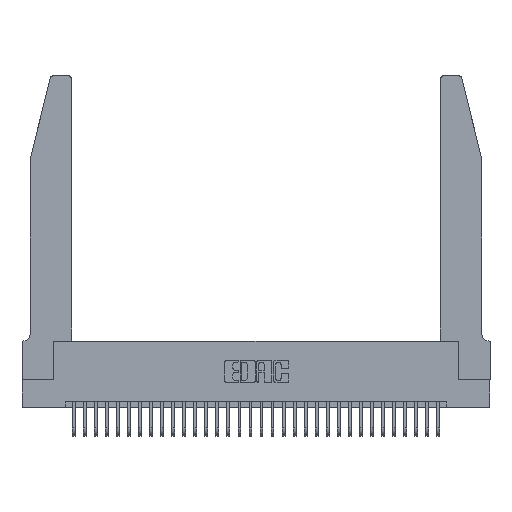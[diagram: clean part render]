
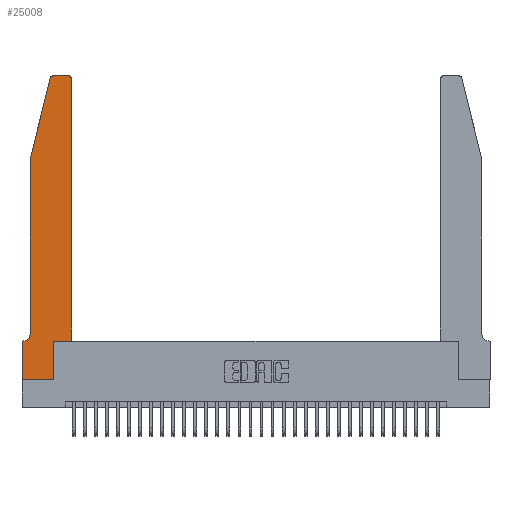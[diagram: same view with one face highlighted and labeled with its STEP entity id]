
A CAD part, top view. The second image highlights one B-rep face of the part: STEP entity #25008.
In plain terms, the highlighted planar face has unit normal (0, 0, 1).
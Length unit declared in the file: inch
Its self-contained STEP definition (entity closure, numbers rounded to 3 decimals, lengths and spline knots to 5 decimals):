
#383 = VECTOR ( 'NONE', #31586, 39.37008 ) ;
#1047 = VECTOR ( 'NONE', #8465, 39.37008 ) ;
#1479 = ORIENTED_EDGE ( 'NONE', *, *, #18732, .T. ) ;
#1792 = CARTESIAN_POINT ( 'NONE',  ( 0.2865, 0.35, 0.37 ) ) ;
#1865 = DIRECTION ( 'NONE',  ( 0., 0., 1. ) ) ;
#2459 = CARTESIAN_POINT ( 'NONE',  ( 0.4205, 2.75, 0.37 ) ) ;
#2580 = VECTOR ( 'NONE', #15802, 39.37008 ) ;
#2673 = ORIENTED_EDGE ( 'NONE', *, *, #33491, .T. ) ;
#2712 = CARTESIAN_POINT ( 'NONE',  ( 0.4505, 0.35, 0.37 ) ) ;
#3021 = CARTESIAN_POINT ( 'NONE',  ( 0.25487, 2.72718, 0.37 ) ) ;
#3065 = ORIENTED_EDGE ( 'NONE', *, *, #3793, .T. ) ;
#3575 = VERTEX_POINT ( 'NONE', #3021 ) ;
#3616 = LINE ( 'NONE', #5594, #4404 ) ;
#3625 = DIRECTION ( 'NONE',  ( 1., 0., 0. ) ) ;
#3793 = EDGE_CURVE ( 'NONE', #13889, #31112, #13183, .T. ) ;
#4172 = CARTESIAN_POINT ( 'NONE',  ( 0.0055, 0.35, 0.37 ) ) ;
#4404 = VECTOR ( 'NONE', #21123, 39.37008 ) ;
#4470 = CARTESIAN_POINT ( 'NONE',  ( 0.2865, 0., 0.37 ) ) ;
#4632 = CARTESIAN_POINT ( 'NONE',  ( 0.284, 2.72, 0.37 ) ) ;
#5594 = CARTESIAN_POINT ( 'NONE',  ( 0.2865, 0.35, 0.37 ) ) ;
#5764 = CIRCLE ( 'NONE', #11834, 0.03 ) ;
#5946 = VECTOR ( 'NONE', #15486, 39.37008 ) ;
#6019 = CARTESIAN_POINT ( 'NONE',  ( 0.2605, 2.75, 0.37 ) ) ;
#6138 = ORIENTED_EDGE ( 'NONE', *, *, #9906, .T. ) ;
#6382 = VECTOR ( 'NONE', #27209, 39.37008 ) ;
#7426 = LINE ( 'NONE', #15679, #383 ) ;
#7627 = ORIENTED_EDGE ( 'NONE', *, *, #19571, .T. ) ;
#7653 = VERTEX_POINT ( 'NONE', #4470 ) ;
#8122 = CARTESIAN_POINT ( 'NONE',  ( 0., 0.35, 0.37 ) ) ;
#8219 = CARTESIAN_POINT ( 'NONE',  ( 0.4205, 2.72, 0.37 ) ) ;
#8465 = DIRECTION ( 'NONE',  ( -1., 0., 0. ) ) ;
#8572 = CARTESIAN_POINT ( 'NONE',  ( 0.0755, 0.42, 0.37 ) ) ;
#9618 = CARTESIAN_POINT ( 'NONE',  ( 0.0755, 0.35, 0.37 ) ) ;
#9860 = DIRECTION ( 'NONE',  ( 1., 0., 0. ) ) ;
#9906 = EDGE_CURVE ( 'NONE', #3575, #31152, #27036, .T. ) ;
#10880 = DIRECTION ( 'NONE',  ( 0., 0., 1. ) ) ;
#11415 = LINE ( 'NONE', #6019, #1047 ) ;
#11450 = VERTEX_POINT ( 'NONE', #1792 ) ;
#11663 = ORIENTED_EDGE ( 'NONE', *, *, #15261, .T. ) ;
#11834 = AXIS2_PLACEMENT_3D ( 'NONE', #8219, #10880, #29340 ) ;
#12582 = ORIENTED_EDGE ( 'NONE', *, *, #31555, .T. ) ;
#13183 = LINE ( 'NONE', #9618, #25977 ) ;
#13426 = CARTESIAN_POINT ( 'NONE',  ( 0.0055, 0.42, 0.37 ) ) ;
#13532 = ORIENTED_EDGE ( 'NONE', *, *, #15069, .T. ) ;
#13828 = VERTEX_POINT ( 'NONE', #19367 ) ;
#13889 = VERTEX_POINT ( 'NONE', #4172 ) ;
#14414 = CARTESIAN_POINT ( 'NONE',  ( 0.0755, 2., 0.37 ) ) ;
#14531 = VECTOR ( 'NONE', #3625, 39.37008 ) ;
#15069 = EDGE_CURVE ( 'NONE', #31152, #25113, #33337, .T. ) ;
#15261 = EDGE_CURVE ( 'NONE', #7653, #11450, #3616, .T. ) ;
#15402 = CIRCLE ( 'NONE', #25035, 0.07 ) ;
#15486 = DIRECTION ( 'NONE',  ( -0.239, -0.971, 0. ) ) ;
#15679 = CARTESIAN_POINT ( 'NONE',  ( 0.4505, 0.35, 0.37 ) ) ;
#15802 = DIRECTION ( 'NONE',  ( 1., 0., 0. ) ) ;
#15987 = AXIS2_PLACEMENT_3D ( 'NONE', #4632, #1865, #9860 ) ;
#16088 = DIRECTION ( 'NONE',  ( 1., 0., 0. ) ) ;
#16699 = CARTESIAN_POINT ( 'NONE',  ( 0., 0., 0.37 ) ) ;
#16907 = CARTESIAN_POINT ( 'NONE',  ( 0.284, 2.75, 0.37 ) ) ;
#17473 = DIRECTION ( 'NONE',  ( -1., 0., 0. ) ) ;
#18188 = ORIENTED_EDGE ( 'NONE', *, *, #27836, .T. ) ;
#18357 = DIRECTION ( 'NONE',  ( 0., -1., 0. ) ) ;
#18454 = EDGE_CURVE ( 'NONE', #29182, #3575, #23302, .T. ) ;
#18732 = EDGE_CURVE ( 'NONE', #25113, #13889, #15402, .T. ) ;
#19367 = CARTESIAN_POINT ( 'NONE',  ( 0.4505, 0.35, 0.37 ) ) ;
#19571 = EDGE_CURVE ( 'NONE', #19877, #7653, #28974, .T. ) ;
#19877 = VERTEX_POINT ( 'NONE', #26173 ) ;
#20504 = EDGE_CURVE ( 'NONE', #31112, #19877, #26648, .T. ) ;
#21123 = DIRECTION ( 'NONE',  ( 0., 1., 0. ) ) ;
#21639 = DIRECTION ( 'NONE',  ( -1., 0., 0. ) ) ;
#22813 = VERTEX_POINT ( 'NONE', #23399 ) ;
#23207 = CARTESIAN_POINT ( 'NONE',  ( 0.0755, 2., 0.37 ) ) ;
#23302 = CIRCLE ( 'NONE', #15987, 0.03 ) ;
#23399 = CARTESIAN_POINT ( 'NONE',  ( 0.4505, 2.72, 0.37 ) ) ;
#23943 = PLANE ( 'NONE',  #31988 ) ;
#24231 = ORIENTED_EDGE ( 'NONE', *, *, #18454, .T. ) ;
#24358 = CARTESIAN_POINT ( 'NONE',  ( 0., 0.35, 0.37 ) ) ;
#24923 = LINE ( 'NONE', #2712, #2580 ) ;
#25008 = ADVANCED_FACE ( 'NONE', ( #28483 ), #23943, .T. ) ;
#25035 = AXIS2_PLACEMENT_3D ( 'NONE', #13426, #29467, #21639 ) ;
#25113 = VERTEX_POINT ( 'NONE', #8572 ) ;
#25977 = VECTOR ( 'NONE', #17473, 39.37008 ) ;
#26173 = CARTESIAN_POINT ( 'NONE',  ( 0., 0., 0.37 ) ) ;
#26598 = DIRECTION ( 'NONE',  ( 0., 0., 1. ) ) ;
#26648 = LINE ( 'NONE', #16699, #6382 ) ;
#27036 = LINE ( 'NONE', #34022, #5946 ) ;
#27062 = ORIENTED_EDGE ( 'NONE', *, *, #20504, .T. ) ;
#27209 = DIRECTION ( 'NONE',  ( 0., -1., 0. ) ) ;
#27535 = VERTEX_POINT ( 'NONE', #2459 ) ;
#27573 = CARTESIAN_POINT ( 'NONE',  ( 0., 0., 0.37 ) ) ;
#27615 = VECTOR ( 'NONE', #18357, 39.37008 ) ;
#27836 = EDGE_CURVE ( 'NONE', #27535, #29182, #11415, .T. ) ;
#28483 = FACE_OUTER_BOUND ( 'NONE', #29527, .T. ) ;
#28974 = LINE ( 'NONE', #27573, #14531 ) ;
#29182 = VERTEX_POINT ( 'NONE', #16907 ) ;
#29340 = DIRECTION ( 'NONE',  ( 1., 0., 0. ) ) ;
#29467 = DIRECTION ( 'NONE',  ( 0., 0., -1. ) ) ;
#29527 = EDGE_LOOP ( 'NONE', ( #18188, #24231, #6138, #13532, #1479, #3065, #27062, #7627, #11663, #32226, #12582, #2673 ) ) ;
#29635 = EDGE_CURVE ( 'NONE', #11450, #13828, #24923, .T. ) ;
#31112 = VERTEX_POINT ( 'NONE', #24358 ) ;
#31152 = VERTEX_POINT ( 'NONE', #14414 ) ;
#31555 = EDGE_CURVE ( 'NONE', #13828, #22813, #7426, .T. ) ;
#31586 = DIRECTION ( 'NONE',  ( 0., 1., 0. ) ) ;
#31988 = AXIS2_PLACEMENT_3D ( 'NONE', #8122, #26598, #16088 ) ;
#32226 = ORIENTED_EDGE ( 'NONE', *, *, #29635, .T. ) ;
#33337 = LINE ( 'NONE', #23207, #27615 ) ;
#33491 = EDGE_CURVE ( 'NONE', #22813, #27535, #5764, .T. ) ;
#34022 = CARTESIAN_POINT ( 'NONE',  ( 0.0755, 2., 0.37 ) ) ;
